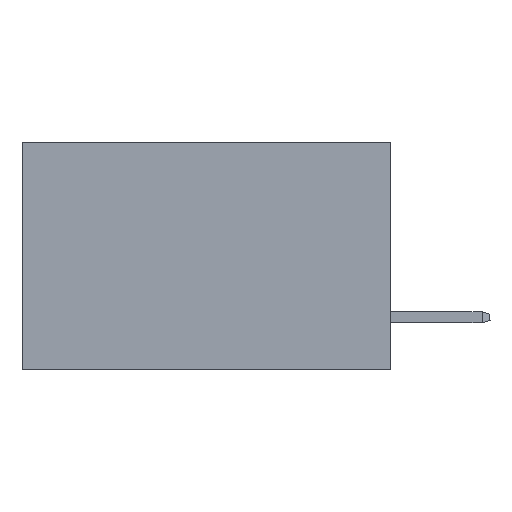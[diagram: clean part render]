
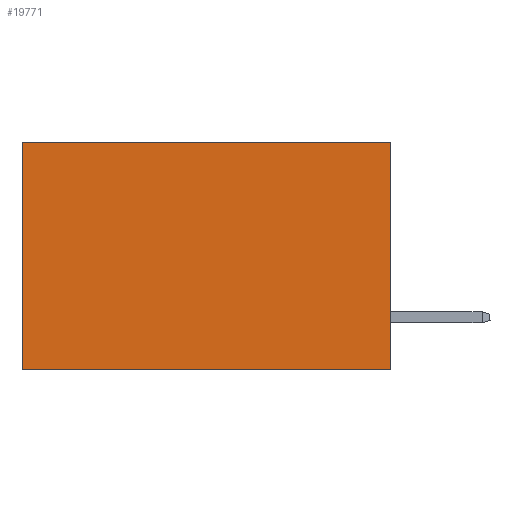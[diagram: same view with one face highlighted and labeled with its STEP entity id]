
A CAD part, left-side view. The second image highlights one B-rep face of the part: STEP entity #19771.
In plain terms, the highlighted planar face has unit normal (-1, 0, 0).
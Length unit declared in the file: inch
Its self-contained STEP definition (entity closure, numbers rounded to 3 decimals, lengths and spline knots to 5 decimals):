
#2036 = DIRECTION ( 'NONE',  ( 0., 1., 0. ) ) ;
#2277 = ORIENTED_EDGE ( 'NONE', *, *, #9920, .T. ) ;
#2411 = CARTESIAN_POINT ( 'NONE',  ( 0.2875, 0.6, -0.37 ) ) ;
#6249 = VECTOR ( 'NONE', #23213, 39.37008 ) ;
#8697 = VERTEX_POINT ( 'NONE', #38768 ) ;
#9920 = EDGE_CURVE ( 'NONE', #8697, #13797, #15577, .T. ) ;
#11707 = EDGE_CURVE ( 'NONE', #24219, #8697, #30472, .T. ) ;
#13677 = CARTESIAN_POINT ( 'NONE',  ( 0.2875, 0., -0.37 ) ) ;
#13797 = VERTEX_POINT ( 'NONE', #2411 ) ;
#14368 = CARTESIAN_POINT ( 'NONE',  ( 0.2875, 0., -0.37 ) ) ;
#14886 = AXIS2_PLACEMENT_3D ( 'NONE', #33871, #36753, #21797 ) ;
#15577 = LINE ( 'NONE', #34738, #6249 ) ;
#16260 = FACE_OUTER_BOUND ( 'NONE', #26498, .T. ) ;
#19771 = ADVANCED_FACE ( 'NONE', ( #16260 ), #37269, .F. ) ;
#21774 = ORIENTED_EDGE ( 'NONE', *, *, #11707, .T. ) ;
#21778 = CARTESIAN_POINT ( 'NONE',  ( 0.2875, 0., 0. ) ) ;
#21797 = DIRECTION ( 'NONE',  ( 0., 0., -1. ) ) ;
#22344 = DIRECTION ( 'NONE',  ( 0., 0., -1. ) ) ;
#23213 = DIRECTION ( 'NONE',  ( 0., 0., -1. ) ) ;
#24219 = VERTEX_POINT ( 'NONE', #21778 ) ;
#24506 = VECTOR ( 'NONE', #22344, 39.37008 ) ;
#25819 = DIRECTION ( 'NONE',  ( 0., 1., 0. ) ) ;
#25960 = VERTEX_POINT ( 'NONE', #14368 ) ;
#26224 = ORIENTED_EDGE ( 'NONE', *, *, #27171, .F. ) ;
#26498 = EDGE_LOOP ( 'NONE', ( #2277, #38363, #26224, #21774 ) ) ;
#27171 = EDGE_CURVE ( 'NONE', #24219, #25960, #33868, .T. ) ;
#27233 = VECTOR ( 'NONE', #25819, 39.37008 ) ;
#27852 = EDGE_CURVE ( 'NONE', #25960, #13797, #33873, .T. ) ;
#28180 = VECTOR ( 'NONE', #2036, 39.37008 ) ;
#28380 = CARTESIAN_POINT ( 'NONE',  ( 0.2875, 0., 0. ) ) ;
#28822 = CARTESIAN_POINT ( 'NONE',  ( 0.2875, 0., 0. ) ) ;
#30472 = LINE ( 'NONE', #28822, #27233 ) ;
#33868 = LINE ( 'NONE', #28380, #24506 ) ;
#33871 = CARTESIAN_POINT ( 'NONE',  ( 0.2875, 0., 0. ) ) ;
#33873 = LINE ( 'NONE', #13677, #28180 ) ;
#34738 = CARTESIAN_POINT ( 'NONE',  ( 0.2875, 0.6, 0. ) ) ;
#36753 = DIRECTION ( 'NONE',  ( 1., 0., 0. ) ) ;
#37269 = PLANE ( 'NONE',  #14886 ) ;
#38363 = ORIENTED_EDGE ( 'NONE', *, *, #27852, .F. ) ;
#38768 = CARTESIAN_POINT ( 'NONE',  ( 0.2875, 0.6, 0. ) ) ;
